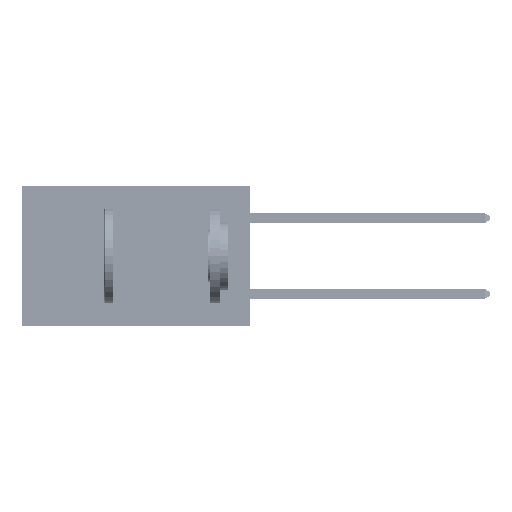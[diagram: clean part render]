
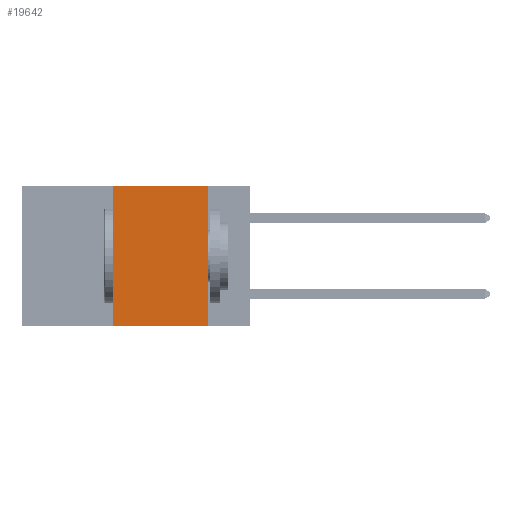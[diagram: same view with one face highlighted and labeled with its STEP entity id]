
A CAD part, left-side view. The second image highlights one B-rep face of the part: STEP entity #19642.
In plain terms, the highlighted planar face has unit normal (-1, 0, 0).
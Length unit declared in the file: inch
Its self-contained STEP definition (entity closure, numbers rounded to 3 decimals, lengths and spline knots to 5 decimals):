
#1514 = EDGE_CURVE ( 'NONE', #14093, #8525, #46476, .T. ) ;
#4729 = EDGE_LOOP ( 'NONE', ( #37240, #25212, #20049, #27239 ) ) ;
#6226 = VECTOR ( 'NONE', #16331, 39.37008 ) ;
#8408 = CARTESIAN_POINT ( 'NONE',  ( 0., 0.11, 0. ) ) ;
#8525 = VERTEX_POINT ( 'NONE', #39833 ) ;
#9148 = EDGE_CURVE ( 'NONE', #14093, #23322, #37706, .T. ) ;
#10610 = VECTOR ( 'NONE', #10721, 39.37008 ) ;
#10721 = DIRECTION ( 'NONE',  ( 0., 0., 1. ) ) ;
#13288 = CARTESIAN_POINT ( 'NONE',  ( 0., 0.36, -0.37 ) ) ;
#14093 = VERTEX_POINT ( 'NONE', #13288 ) ;
#15575 = EDGE_CURVE ( 'NONE', #23322, #40227, #21563, .T. ) ;
#16108 = AXIS2_PLACEMENT_3D ( 'NONE', #17589, #46037, #24399 ) ;
#16331 = DIRECTION ( 'NONE',  ( 0., 0., -1. ) ) ;
#17589 = CARTESIAN_POINT ( 'NONE',  ( 0., 0.6, 0. ) ) ;
#17726 = CARTESIAN_POINT ( 'NONE',  ( 0., 0.6, -0.37 ) ) ;
#19642 = ADVANCED_FACE ( 'NONE', ( #35451 ), #38892, .F. ) ;
#20049 = ORIENTED_EDGE ( 'NONE', *, *, #9148, .F. ) ;
#21563 = LINE ( 'NONE', #41141, #36217 ) ;
#23322 = VERTEX_POINT ( 'NONE', #36734 ) ;
#24399 = DIRECTION ( 'NONE',  ( 0., 0., -1. ) ) ;
#25212 = ORIENTED_EDGE ( 'NONE', *, *, #15575, .F. ) ;
#27239 = ORIENTED_EDGE ( 'NONE', *, *, #1514, .T. ) ;
#27447 = CARTESIAN_POINT ( 'NONE',  ( 0., 0.11, 0. ) ) ;
#28629 = DIRECTION ( 'NONE',  ( 0., -1., 0. ) ) ;
#30572 = LINE ( 'NONE', #8408, #6226 ) ;
#32508 = CARTESIAN_POINT ( 'NONE',  ( 0., 0.36, 0. ) ) ;
#33172 = EDGE_CURVE ( 'NONE', #40227, #8525, #30572, .T. ) ;
#34749 = DIRECTION ( 'NONE',  ( 0., -1., 0. ) ) ;
#35451 = FACE_OUTER_BOUND ( 'NONE', #4729, .T. ) ;
#35712 = VECTOR ( 'NONE', #28629, 39.37008 ) ;
#36217 = VECTOR ( 'NONE', #34749, 39.37008 ) ;
#36734 = CARTESIAN_POINT ( 'NONE',  ( 0., 0.36, 0. ) ) ;
#37240 = ORIENTED_EDGE ( 'NONE', *, *, #33172, .F. ) ;
#37706 = LINE ( 'NONE', #32508, #10610 ) ;
#38892 = PLANE ( 'NONE',  #16108 ) ;
#39833 = CARTESIAN_POINT ( 'NONE',  ( 0., 0.11, -0.37 ) ) ;
#40227 = VERTEX_POINT ( 'NONE', #27447 ) ;
#41141 = CARTESIAN_POINT ( 'NONE',  ( 0., 0.6, 0. ) ) ;
#46037 = DIRECTION ( 'NONE',  ( 1., 0., 0. ) ) ;
#46476 = LINE ( 'NONE', #17726, #35712 ) ;
